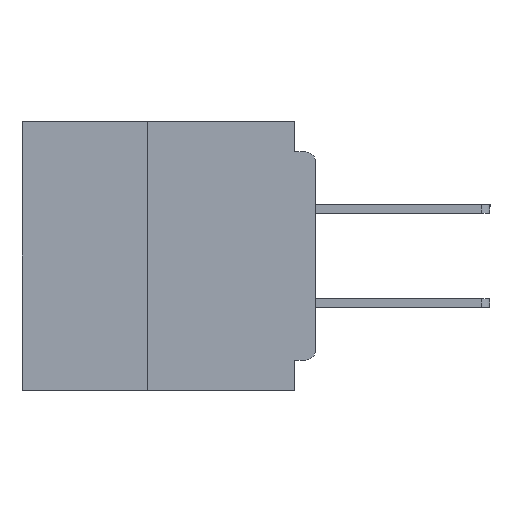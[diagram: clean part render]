
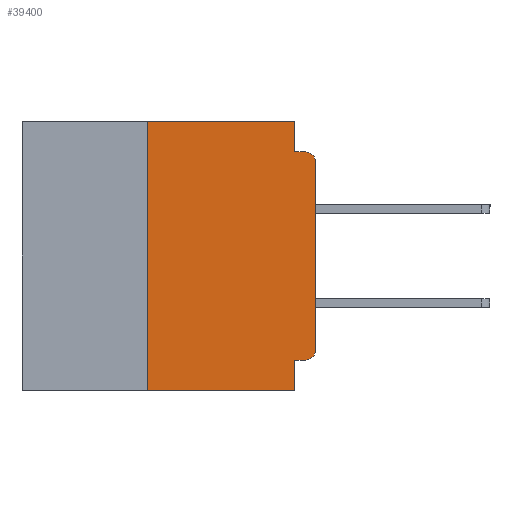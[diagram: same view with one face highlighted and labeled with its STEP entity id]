
A CAD part, left-side view. The second image highlights one B-rep face of the part: STEP entity #39400.
In plain terms, the highlighted planar face has unit normal (-1, 0, 0).
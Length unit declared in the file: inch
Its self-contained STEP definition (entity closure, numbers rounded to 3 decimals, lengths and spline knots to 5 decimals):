
#571 = EDGE_CURVE ( 'NONE', #40105, #4981, #17307, .T. ) ;
#1060 = EDGE_CURVE ( 'NONE', #13123, #35625, #29610, .T. ) ;
#1508 = VECTOR ( 'NONE', #32934, 39.37008 ) ;
#1599 = CIRCLE ( 'NONE', #12824, 0.015 ) ;
#1717 = DIRECTION ( 'NONE',  ( 0., 0., -1. ) ) ;
#2344 = CARTESIAN_POINT ( 'NONE',  ( 0., 0., -0.045 ) ) ;
#2979 = DIRECTION ( 'NONE',  ( 0., 0., 1. ) ) ;
#4918 = LINE ( 'NONE', #15832, #59127 ) ;
#4981 = VERTEX_POINT ( 'NONE', #64676 ) ;
#5195 = CARTESIAN_POINT ( 'NONE',  ( 0., 0., -0.355 ) ) ;
#5361 = DIRECTION ( 'NONE',  ( 0., 1., 0. ) ) ;
#6591 = VERTEX_POINT ( 'NONE', #20290 ) ;
#6941 = VERTEX_POINT ( 'NONE', #64878 ) ;
#7479 = LINE ( 'NONE', #9237, #44457 ) ;
#7662 = DIRECTION ( 'NONE',  ( 0., -1., 0. ) ) ;
#7731 = DIRECTION ( 'NONE',  ( 1., 0., 0. ) ) ;
#9237 = CARTESIAN_POINT ( 'NONE',  ( 0., 0.437, 0. ) ) ;
#11587 = CARTESIAN_POINT ( 'NONE',  ( 0., 0.015, -0.06 ) ) ;
#11614 = DIRECTION ( 'NONE',  ( 0., 0., -1. ) ) ;
#11686 = EDGE_CURVE ( 'NONE', #45039, #50701, #17972, .T. ) ;
#12824 = AXIS2_PLACEMENT_3D ( 'NONE', #64637, #33328, #1717 ) ;
#13123 = VERTEX_POINT ( 'NONE', #49709 ) ;
#13973 = VECTOR ( 'NONE', #22470, 39.37008 ) ;
#15626 = LINE ( 'NONE', #43354, #13973 ) ;
#15756 = CARTESIAN_POINT ( 'NONE',  ( 0., 0.015, -0.045 ) ) ;
#15832 = CARTESIAN_POINT ( 'NONE',  ( 0., 0.031, -0.4 ) ) ;
#16070 = VECTOR ( 'NONE', #7662, 39.37008 ) ;
#16917 = DIRECTION ( 'NONE',  ( 0., 0., -1. ) ) ;
#17307 = LINE ( 'NONE', #5195, #57491 ) ;
#17972 = CIRCLE ( 'NONE', #54915, 0.015 ) ;
#18257 = CARTESIAN_POINT ( 'NONE',  ( 0., 0.031, -0.4 ) ) ;
#20290 = CARTESIAN_POINT ( 'NONE',  ( 0., 0., -0.34 ) ) ;
#20719 = EDGE_LOOP ( 'NONE', ( #27375, #36132, #47352, #45712, #57056, #30800, #49641, #45919, #23888, #46666 ) ) ;
#21164 = DIRECTION ( 'NONE',  ( 0., 0., -1. ) ) ;
#22470 = DIRECTION ( 'NONE',  ( 0., -1., 0. ) ) ;
#23888 = ORIENTED_EDGE ( 'NONE', *, *, #571, .F. ) ;
#24017 = EDGE_CURVE ( 'NONE', #40105, #6591, #1599, .T. ) ;
#24190 = VECTOR ( 'NONE', #2979, 39.37008 ) ;
#25242 = AXIS2_PLACEMENT_3D ( 'NONE', #39232, #7731, #44485 ) ;
#25822 = VERTEX_POINT ( 'NONE', #18257 ) ;
#27375 = ORIENTED_EDGE ( 'NONE', *, *, #66771, .T. ) ;
#28854 = CARTESIAN_POINT ( 'NONE',  ( 0., 0.25, 0. ) ) ;
#28953 = CARTESIAN_POINT ( 'NONE',  ( 0., 0.015, -0.355 ) ) ;
#29610 = LINE ( 'NONE', #33057, #1508 ) ;
#30127 = LINE ( 'NONE', #2344, #16070 ) ;
#30800 = ORIENTED_EDGE ( 'NONE', *, *, #1060, .F. ) ;
#32934 = DIRECTION ( 'NONE',  ( 0., 0., 1. ) ) ;
#33057 = CARTESIAN_POINT ( 'NONE',  ( 0., 0.25, -0.4 ) ) ;
#33328 = DIRECTION ( 'NONE',  ( -1., 0., 0. ) ) ;
#33613 = EDGE_CURVE ( 'NONE', #35625, #45469, #7479, .T. ) ;
#34186 = CARTESIAN_POINT ( 'NONE',  ( 0., 0.031, 0. ) ) ;
#34741 = VECTOR ( 'NONE', #11614, 39.37008 ) ;
#35002 = EDGE_CURVE ( 'NONE', #13123, #25822, #15626, .T. ) ;
#35625 = VERTEX_POINT ( 'NONE', #28854 ) ;
#36132 = ORIENTED_EDGE ( 'NONE', *, *, #11686, .T. ) ;
#39088 = EDGE_CURVE ( 'NONE', #4981, #25822, #4918, .T. ) ;
#39232 = CARTESIAN_POINT ( 'NONE',  ( 0., 0.437, 0. ) ) ;
#39400 = ADVANCED_FACE ( 'NONE', ( #50037 ), #65304, .F. ) ;
#40105 = VERTEX_POINT ( 'NONE', #28953 ) ;
#42600 = EDGE_CURVE ( 'NONE', #6941, #50701, #30127, .T. ) ;
#43354 = CARTESIAN_POINT ( 'NONE',  ( 0., 0.437, -0.4 ) ) ;
#44457 = VECTOR ( 'NONE', #51235, 39.37008 ) ;
#44485 = DIRECTION ( 'NONE',  ( 0., 0., -1. ) ) ;
#45039 = VERTEX_POINT ( 'NONE', #56670 ) ;
#45469 = VERTEX_POINT ( 'NONE', #34186 ) ;
#45712 = ORIENTED_EDGE ( 'NONE', *, *, #67741, .F. ) ;
#45919 = ORIENTED_EDGE ( 'NONE', *, *, #39088, .F. ) ;
#46666 = ORIENTED_EDGE ( 'NONE', *, *, #24017, .T. ) ;
#46976 = LINE ( 'NONE', #58879, #34741 ) ;
#47352 = ORIENTED_EDGE ( 'NONE', *, *, #42600, .F. ) ;
#48302 = DIRECTION ( 'NONE',  ( -1., 0., 0. ) ) ;
#49641 = ORIENTED_EDGE ( 'NONE', *, *, #35002, .T. ) ;
#49709 = CARTESIAN_POINT ( 'NONE',  ( 0., 0.25, -0.4 ) ) ;
#50037 = FACE_OUTER_BOUND ( 'NONE', #20719, .T. ) ;
#50701 = VERTEX_POINT ( 'NONE', #15756 ) ;
#51235 = DIRECTION ( 'NONE',  ( 0., -1., 0. ) ) ;
#54915 = AXIS2_PLACEMENT_3D ( 'NONE', #11587, #48302, #16917 ) ;
#56670 = CARTESIAN_POINT ( 'NONE',  ( 0., 0., -0.06 ) ) ;
#57056 = ORIENTED_EDGE ( 'NONE', *, *, #33613, .F. ) ;
#57491 = VECTOR ( 'NONE', #5361, 39.37008 ) ;
#58879 = CARTESIAN_POINT ( 'NONE',  ( 0., 0.031, 0. ) ) ;
#59127 = VECTOR ( 'NONE', #21164, 39.37008 ) ;
#64637 = CARTESIAN_POINT ( 'NONE',  ( 0., 0.015, -0.34 ) ) ;
#64676 = CARTESIAN_POINT ( 'NONE',  ( 0., 0.031, -0.355 ) ) ;
#64878 = CARTESIAN_POINT ( 'NONE',  ( 0., 0.031, -0.045 ) ) ;
#65304 = PLANE ( 'NONE',  #25242 ) ;
#65856 = CARTESIAN_POINT ( 'NONE',  ( 0., 0., 0. ) ) ;
#65971 = LINE ( 'NONE', #65856, #24190 ) ;
#66771 = EDGE_CURVE ( 'NONE', #6591, #45039, #65971, .T. ) ;
#67741 = EDGE_CURVE ( 'NONE', #45469, #6941, #46976, .T. ) ;
